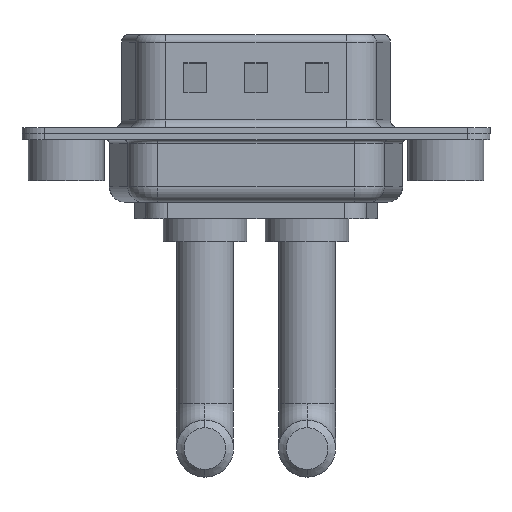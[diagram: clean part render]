
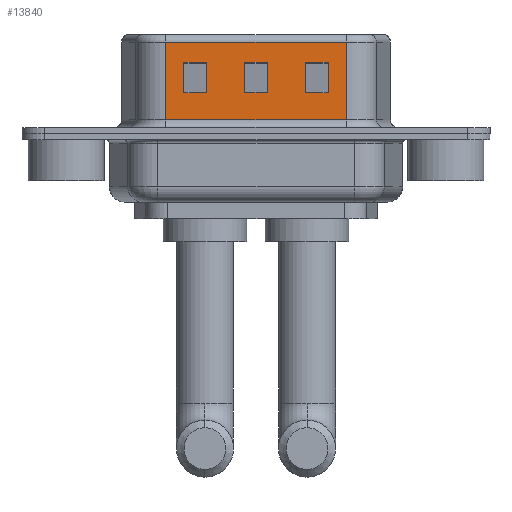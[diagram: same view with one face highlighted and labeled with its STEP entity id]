
A CAD part, front view. The second image highlights one B-rep face of the part: STEP entity #13840.
In plain terms, the highlighted planar face has unit normal (0, -1, 0).
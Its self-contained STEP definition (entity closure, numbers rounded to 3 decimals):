
#30 = ORIENTED_EDGE ( 'NONE', *, *, #13751, .T. ) ;
#109 = DIRECTION ( 'NONE',  ( 0., 0., 1. ) ) ;
#241 = CARTESIAN_POINT ( 'NONE',  ( 13.25, -4.55, 6.52 ) ) ;
#328 = LINE ( 'NONE', #5011, #8408 ) ;
#360 = CARTESIAN_POINT ( 'NONE',  ( 22.451, -4.55, 4.705 ) ) ;
#467 = CARTESIAN_POINT ( 'NONE',  ( 6.549, -4.55, 0.9 ) ) ;
#589 = VERTEX_POINT ( 'NONE', #5961 ) ;
#750 = FACE_BOUND ( 'NONE', #5758, .T. ) ;
#841 = LINE ( 'NONE', #4423, #10835 ) ;
#914 = ORIENTED_EDGE ( 'NONE', *, *, #7913, .T. ) ;
#916 = LINE ( 'NONE', #8707, #7139 ) ;
#921 = VECTOR ( 'NONE', #14411, 1000. ) ;
#984 = VERTEX_POINT ( 'NONE', #7977 ) ;
#1133 = LINE ( 'NONE', #2221, #8630 ) ;
#1317 = LINE ( 'NONE', #9252, #1912 ) ;
#1421 = ORIENTED_EDGE ( 'NONE', *, *, #13080, .T. ) ;
#1469 = EDGE_CURVE ( 'NONE', #6099, #6190, #1317, .T. ) ;
#1523 = DIRECTION ( 'NONE',  ( 0., 0., -1. ) ) ;
#1553 = EDGE_CURVE ( 'NONE', #9471, #13779, #13608, .T. ) ;
#1598 = CARTESIAN_POINT ( 'NONE',  ( 17.25, -4.55, 6.52 ) ) ;
#1673 = EDGE_LOOP ( 'NONE', ( #2886, #4013, #12360, #8340 ) ) ;
#1805 = CARTESIAN_POINT ( 'NONE',  ( 6.549, -4.55, 6.52 ) ) ;
#1907 = DIRECTION ( 'NONE',  ( -1., 0., 0. ) ) ;
#1912 = VECTOR ( 'NONE', #9180, 1000. ) ;
#1951 = ORIENTED_EDGE ( 'NONE', *, *, #10798, .T. ) ;
#2193 = EDGE_CURVE ( 'NONE', #7781, #7983, #6135, .T. ) ;
#2221 = CARTESIAN_POINT ( 'NONE',  ( 7.75, -4.55, 6.52 ) ) ;
#2502 = CARTESIAN_POINT ( 'NONE',  ( 18.451, -4.55, 4.705 ) ) ;
#2585 = CARTESIAN_POINT ( 'NONE',  ( 22.451, -4.55, 2.705 ) ) ;
#2589 = DIRECTION ( 'NONE',  ( 0., 0., -1. ) ) ;
#2886 = ORIENTED_EDGE ( 'NONE', *, *, #14240, .T. ) ;
#3020 = CARTESIAN_POINT ( 'NONE',  ( 15.75, -4.55, 2.705 ) ) ;
#3069 = VECTOR ( 'NONE', #13621, 1000. ) ;
#3070 = DIRECTION ( 'NONE',  ( -1., 0., 0. ) ) ;
#3106 = EDGE_CURVE ( 'NONE', #6671, #10922, #3699, .T. ) ;
#3367 = EDGE_LOOP ( 'NONE', ( #914, #30, #3910, #6299 ) ) ;
#3375 = CARTESIAN_POINT ( 'NONE',  ( 15.75, -4.55, 4.705 ) ) ;
#3699 = LINE ( 'NONE', #8150, #12177 ) ;
#3910 = ORIENTED_EDGE ( 'NONE', *, *, #6297, .T. ) ;
#4013 = ORIENTED_EDGE ( 'NONE', *, *, #11808, .T. ) ;
#4200 = CARTESIAN_POINT ( 'NONE',  ( 11.75, -4.55, 6.52 ) ) ;
#4245 = VECTOR ( 'NONE', #11837, 1000. ) ;
#4326 = VERTEX_POINT ( 'NONE', #10913 ) ;
#4423 = CARTESIAN_POINT ( 'NONE',  ( 18.451, -4.55, 6.02 ) ) ;
#4702 = VECTOR ( 'NONE', #6350, 1000. ) ;
#4995 = CARTESIAN_POINT ( 'NONE',  ( 17.25, -4.55, 2.705 ) ) ;
#5011 = CARTESIAN_POINT ( 'NONE',  ( 9.25, -4.55, 6.52 ) ) ;
#5187 = CARTESIAN_POINT ( 'NONE',  ( 7.75, -4.55, 2.705 ) ) ;
#5278 = PLANE ( 'NONE',  #7269 ) ;
#5284 = ORIENTED_EDGE ( 'NONE', *, *, #6307, .T. ) ;
#5331 = VECTOR ( 'NONE', #7039, 1000. ) ;
#5758 = EDGE_LOOP ( 'NONE', ( #10797, #9984, #1421, #10598 ) ) ;
#5864 = ORIENTED_EDGE ( 'NONE', *, *, #2193, .T. ) ;
#5961 = CARTESIAN_POINT ( 'NONE',  ( 13.25, -4.55, 4.705 ) ) ;
#6099 = VERTEX_POINT ( 'NONE', #11590 ) ;
#6135 = LINE ( 'NONE', #1805, #4702 ) ;
#6163 = FACE_BOUND ( 'NONE', #3367, .T. ) ;
#6190 = VERTEX_POINT ( 'NONE', #11659 ) ;
#6293 = LINE ( 'NONE', #1598, #4245 ) ;
#6297 = EDGE_CURVE ( 'NONE', #10055, #984, #916, .T. ) ;
#6299 = ORIENTED_EDGE ( 'NONE', *, *, #10248, .T. ) ;
#6307 = EDGE_CURVE ( 'NONE', #9471, #7781, #841, .T. ) ;
#6350 = DIRECTION ( 'NONE',  ( 0., 0., -1. ) ) ;
#6368 = ORIENTED_EDGE ( 'NONE', *, *, #1553, .F. ) ;
#6370 = LINE ( 'NONE', #8675, #8773 ) ;
#6466 = DIRECTION ( 'NONE',  ( 0., 0., 1. ) ) ;
#6558 = CARTESIAN_POINT ( 'NONE',  ( 6.549, -4.55, 6.02 ) ) ;
#6671 = VERTEX_POINT ( 'NONE', #3020 ) ;
#7039 = DIRECTION ( 'NONE',  ( 1., 0., 0. ) ) ;
#7094 = LINE ( 'NONE', #241, #3069 ) ;
#7105 = LINE ( 'NONE', #2502, #5331 ) ;
#7139 = VECTOR ( 'NONE', #12084, 1000. ) ;
#7142 = LINE ( 'NONE', #360, #11318 ) ;
#7162 = EDGE_CURVE ( 'NONE', #14186, #7766, #6370, .T. ) ;
#7269 = AXIS2_PLACEMENT_3D ( 'NONE', #10776, #11856, #1907 ) ;
#7412 = EDGE_LOOP ( 'NONE', ( #6368, #5284, #5864, #1951 ) ) ;
#7766 = VERTEX_POINT ( 'NONE', #5187 ) ;
#7781 = VERTEX_POINT ( 'NONE', #6558 ) ;
#7880 = VECTOR ( 'NONE', #6466, 1000. ) ;
#7905 = DIRECTION ( 'NONE',  ( 1., 0., 0. ) ) ;
#7913 = EDGE_CURVE ( 'NONE', #4326, #589, #7105, .T. ) ;
#7977 = CARTESIAN_POINT ( 'NONE',  ( 11.75, -4.55, 2.705 ) ) ;
#7983 = VERTEX_POINT ( 'NONE', #467 ) ;
#8150 = CARTESIAN_POINT ( 'NONE',  ( 15.75, -4.55, 6.52 ) ) ;
#8185 = EDGE_CURVE ( 'NONE', #10922, #14307, #7142, .T. ) ;
#8222 = CARTESIAN_POINT ( 'NONE',  ( 13.25, -4.55, 2.705 ) ) ;
#8320 = CARTESIAN_POINT ( 'NONE',  ( 18.451, -4.55, 6.52 ) ) ;
#8334 = FACE_OUTER_BOUND ( 'NONE', #7412, .T. ) ;
#8340 = ORIENTED_EDGE ( 'NONE', *, *, #8185, .T. ) ;
#8408 = VECTOR ( 'NONE', #2589, 1000. ) ;
#8523 = CARTESIAN_POINT ( 'NONE',  ( 17.25, -4.55, 4.705 ) ) ;
#8630 = VECTOR ( 'NONE', #109, 1000. ) ;
#8675 = CARTESIAN_POINT ( 'NONE',  ( 14.451, -4.55, 2.705 ) ) ;
#8707 = CARTESIAN_POINT ( 'NONE',  ( 18.451, -4.55, 2.705 ) ) ;
#8773 = VECTOR ( 'NONE', #3070, 1000. ) ;
#9180 = DIRECTION ( 'NONE',  ( 1., 0., 0. ) ) ;
#9241 = DIRECTION ( 'NONE',  ( 1., 0., 0. ) ) ;
#9252 = CARTESIAN_POINT ( 'NONE',  ( 14.451, -4.55, 4.705 ) ) ;
#9471 = VERTEX_POINT ( 'NONE', #11333 ) ;
#9624 = CARTESIAN_POINT ( 'NONE',  ( 18.451, -4.55, 0.9 ) ) ;
#9984 = ORIENTED_EDGE ( 'NONE', *, *, #7162, .T. ) ;
#10055 = VERTEX_POINT ( 'NONE', #8222 ) ;
#10248 = EDGE_CURVE ( 'NONE', #984, #4326, #14169, .T. ) ;
#10273 = CARTESIAN_POINT ( 'NONE',  ( 18.451, -4.55, 0.9 ) ) ;
#10509 = VECTOR ( 'NONE', #1523, 1000. ) ;
#10598 = ORIENTED_EDGE ( 'NONE', *, *, #1469, .T. ) ;
#10776 = CARTESIAN_POINT ( 'NONE',  ( 18.451, -4.55, 6.52 ) ) ;
#10797 = ORIENTED_EDGE ( 'NONE', *, *, #13213, .T. ) ;
#10798 = EDGE_CURVE ( 'NONE', #7983, #13779, #12302, .T. ) ;
#10835 = VECTOR ( 'NONE', #14382, 1000. ) ;
#10878 = VECTOR ( 'NONE', #7905, 1000. ) ;
#10913 = CARTESIAN_POINT ( 'NONE',  ( 11.75, -4.55, 4.705 ) ) ;
#10922 = VERTEX_POINT ( 'NONE', #3375 ) ;
#11264 = CARTESIAN_POINT ( 'NONE',  ( 9.25, -4.55, 2.705 ) ) ;
#11318 = VECTOR ( 'NONE', #9241, 1000. ) ;
#11333 = CARTESIAN_POINT ( 'NONE',  ( 18.451, -4.55, 6.02 ) ) ;
#11590 = CARTESIAN_POINT ( 'NONE',  ( 7.75, -4.55, 4.705 ) ) ;
#11659 = CARTESIAN_POINT ( 'NONE',  ( 9.25, -4.55, 4.705 ) ) ;
#11784 = FACE_BOUND ( 'NONE', #1673, .T. ) ;
#11808 = EDGE_CURVE ( 'NONE', #13794, #6671, #12538, .T. ) ;
#11837 = DIRECTION ( 'NONE',  ( 0., 0., -1. ) ) ;
#11856 = DIRECTION ( 'NONE',  ( 0., 1., 0. ) ) ;
#12084 = DIRECTION ( 'NONE',  ( -1., 0., 0. ) ) ;
#12177 = VECTOR ( 'NONE', #12553, 1000. ) ;
#12302 = LINE ( 'NONE', #10273, #10878 ) ;
#12360 = ORIENTED_EDGE ( 'NONE', *, *, #3106, .T. ) ;
#12538 = LINE ( 'NONE', #2585, #921 ) ;
#12553 = DIRECTION ( 'NONE',  ( 0., 0., 1. ) ) ;
#13080 = EDGE_CURVE ( 'NONE', #7766, #6099, #1133, .T. ) ;
#13213 = EDGE_CURVE ( 'NONE', #6190, #14186, #328, .T. ) ;
#13608 = LINE ( 'NONE', #8320, #10509 ) ;
#13621 = DIRECTION ( 'NONE',  ( 0., 0., -1. ) ) ;
#13751 = EDGE_CURVE ( 'NONE', #589, #10055, #7094, .T. ) ;
#13779 = VERTEX_POINT ( 'NONE', #9624 ) ;
#13794 = VERTEX_POINT ( 'NONE', #4995 ) ;
#13840 = ADVANCED_FACE ( 'NONE', ( #750, #11784, #6163, #8334 ), #5278, .F. ) ;
#14169 = LINE ( 'NONE', #4200, #7880 ) ;
#14186 = VERTEX_POINT ( 'NONE', #11264 ) ;
#14240 = EDGE_CURVE ( 'NONE', #14307, #13794, #6293, .T. ) ;
#14307 = VERTEX_POINT ( 'NONE', #8523 ) ;
#14382 = DIRECTION ( 'NONE',  ( -1., 0., 0. ) ) ;
#14411 = DIRECTION ( 'NONE',  ( -1., 0., 0. ) ) ;
